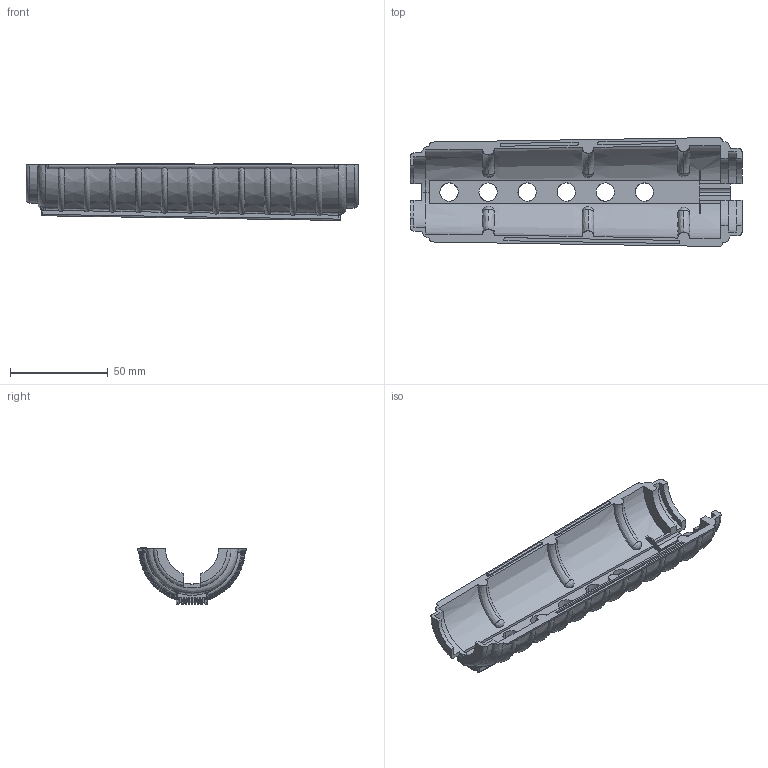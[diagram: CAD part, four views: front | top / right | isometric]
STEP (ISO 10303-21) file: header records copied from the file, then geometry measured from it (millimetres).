
FILE_DESCRIPTION (( 'STEP AP214' ), '1' );
FILE_NAME ('M4-handguard half.STEP', '2013-06-18T15:31:51', ( 'Asher' ), ( '' ), 'SwSTEP 2.0', 'SolidWorks 2013', '' );
FILE_SCHEMA (( 'AUTOMOTIVE_DESIGN' ));
Length unit declared in the file: millimetre
Products named in the file (1): M4-handguard half
Bounding box: 170 x 55.82 x 29.15 mm (x, y, z)
Volume: 36406.7 mm3; surface area: 33345.9 mm2
Topology: 1 solids, 1 shells, 453 faces, 1312 edges, 846 vertices
Faces by surface type: plane 212, cylinder 120, bspline 92, cone 29
Entity records: 21493 total; most frequent: CARTESIAN_POINT 10922, ORIENTED_EDGE 2600, DIRECTION 1715, EDGE_CURVE 1300, VERTEX_POINT 846, LINE 653, VECTOR 653, AXIS2_PLACEMENT_3D 531
